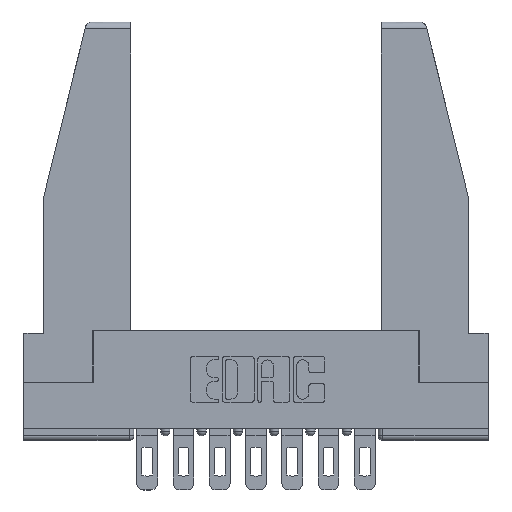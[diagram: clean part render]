
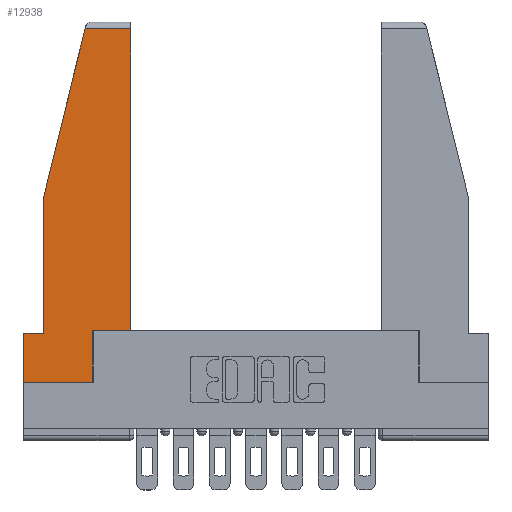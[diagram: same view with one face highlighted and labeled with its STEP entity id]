
A CAD part, top view. The second image highlights one B-rep face of the part: STEP entity #12938.
In plain terms, the highlighted planar face has unit normal (0, 0, 1).
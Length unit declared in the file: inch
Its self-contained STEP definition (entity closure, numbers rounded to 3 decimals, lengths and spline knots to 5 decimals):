
#325 = LINE ( 'NONE', #12492, #6050 ) ;
#330 = EDGE_CURVE ( 'NONE', #11068, #5160, #11624, .T. ) ;
#510 = ORIENTED_EDGE ( 'NONE', *, *, #4445, .T. ) ;
#1410 = LINE ( 'NONE', #4657, #11373 ) ;
#1658 = CARTESIAN_POINT ( 'NONE',  ( 0., 0.21, 0. ) ) ;
#1961 = VERTEX_POINT ( 'NONE', #8863 ) ;
#2006 = DIRECTION ( 'NONE',  ( -0.239, -0.971, 0. ) ) ;
#2107 = DIRECTION ( 'NONE',  ( 0., -1., 0. ) ) ;
#2191 = CARTESIAN_POINT ( 'NONE',  ( 0.086, 0.8, 0. ) ) ;
#2214 = LINE ( 'NONE', #5121, #5008 ) ;
#2404 = EDGE_CURVE ( 'NONE', #5160, #3727, #9088, .T. ) ;
#2433 = VECTOR ( 'NONE', #8961, 39.37008 ) ;
#2549 = CARTESIAN_POINT ( 'NONE',  ( 0.461, 1.52, 0. ) ) ;
#2828 = EDGE_CURVE ( 'NONE', #8333, #1961, #1410, .T. ) ;
#2837 = AXIS2_PLACEMENT_3D ( 'NONE', #11134, #10031, #13263 ) ;
#2905 = DIRECTION ( 'NONE',  ( -1., 0., 0. ) ) ;
#2972 = EDGE_CURVE ( 'NONE', #5855, #11068, #2214, .T. ) ;
#3239 = DIRECTION ( 'NONE',  ( 0., 1., 0. ) ) ;
#3332 = LINE ( 'NONE', #4401, #3661 ) ;
#3661 = VECTOR ( 'NONE', #3239, 39.37008 ) ;
#3727 = VERTEX_POINT ( 'NONE', #4816 ) ;
#3913 = EDGE_CURVE ( 'NONE', #1961, #5855, #3332, .T. ) ;
#4401 = CARTESIAN_POINT ( 'NONE',  ( 0.297, 0., 0. ) ) ;
#4445 = EDGE_CURVE ( 'NONE', #9360, #13013, #13496, .T. ) ;
#4657 = CARTESIAN_POINT ( 'NONE',  ( 0., 0., 0. ) ) ;
#4816 = CARTESIAN_POINT ( 'NONE',  ( 0.2636, 1.52, 0. ) ) ;
#4980 = DIRECTION ( 'NONE',  ( 1., 0., 0. ) ) ;
#5008 = VECTOR ( 'NONE', #4980, 39.37008 ) ;
#5121 = CARTESIAN_POINT ( 'NONE',  ( 0.297, 0.223, 0. ) ) ;
#5160 = VERTEX_POINT ( 'NONE', #2549 ) ;
#5519 = VECTOR ( 'NONE', #2905, 39.37008 ) ;
#5855 = VERTEX_POINT ( 'NONE', #6613 ) ;
#6015 = EDGE_CURVE ( 'NONE', #13013, #8176, #325, .T. ) ;
#6029 = CARTESIAN_POINT ( 'NONE',  ( 0.086, 0.21, 0. ) ) ;
#6050 = VECTOR ( 'NONE', #10335, 39.37008 ) ;
#6460 = EDGE_CURVE ( 'NONE', #8176, #8333, #8006, .T. ) ;
#6544 = ORIENTED_EDGE ( 'NONE', *, *, #6015, .T. ) ;
#6613 = CARTESIAN_POINT ( 'NONE',  ( 0.297, 0.223, 0. ) ) ;
#6689 = EDGE_CURVE ( 'NONE', #3727, #9360, #11585, .T. ) ;
#6868 = PLANE ( 'NONE',  #2837 ) ;
#7839 = EDGE_LOOP ( 'NONE', ( #8641, #9992, #8361, #510, #6544, #10832, #12906, #13343, #13008 ) ) ;
#8006 = LINE ( 'NONE', #1658, #2433 ) ;
#8176 = VERTEX_POINT ( 'NONE', #8384 ) ;
#8222 = FACE_OUTER_BOUND ( 'NONE', #7839, .T. ) ;
#8333 = VERTEX_POINT ( 'NONE', #9545 ) ;
#8361 = ORIENTED_EDGE ( 'NONE', *, *, #6689, .T. ) ;
#8384 = CARTESIAN_POINT ( 'NONE',  ( 0., 0.21, 0. ) ) ;
#8641 = ORIENTED_EDGE ( 'NONE', *, *, #330, .T. ) ;
#8863 = CARTESIAN_POINT ( 'NONE',  ( 0.297, 0., 0. ) ) ;
#8961 = DIRECTION ( 'NONE',  ( 0., -1., 0. ) ) ;
#9088 = LINE ( 'NONE', #9269, #5519 ) ;
#9269 = CARTESIAN_POINT ( 'NONE',  ( 0., 1.52, 0. ) ) ;
#9360 = VERTEX_POINT ( 'NONE', #9475 ) ;
#9475 = CARTESIAN_POINT ( 'NONE',  ( 0.086, 0.8, 0. ) ) ;
#9545 = CARTESIAN_POINT ( 'NONE',  ( 0., 0., 0. ) ) ;
#9992 = ORIENTED_EDGE ( 'NONE', *, *, #2404, .T. ) ;
#10031 = DIRECTION ( 'NONE',  ( 0., 0., 1. ) ) ;
#10335 = DIRECTION ( 'NONE',  ( -1., 0., 0. ) ) ;
#10365 = VECTOR ( 'NONE', #2107, 39.37008 ) ;
#10469 = CARTESIAN_POINT ( 'NONE',  ( 0.271, 1.55, 0. ) ) ;
#10832 = ORIENTED_EDGE ( 'NONE', *, *, #6460, .T. ) ;
#11015 = DIRECTION ( 'NONE',  ( 0., 1., 0. ) ) ;
#11068 = VERTEX_POINT ( 'NONE', #11638 ) ;
#11108 = VECTOR ( 'NONE', #11015, 39.37008 ) ;
#11134 = CARTESIAN_POINT ( 'NONE',  ( 0., 0., 0. ) ) ;
#11373 = VECTOR ( 'NONE', #12001, 39.37008 ) ;
#11585 = LINE ( 'NONE', #10469, #11905 ) ;
#11624 = LINE ( 'NONE', #12032, #11108 ) ;
#11638 = CARTESIAN_POINT ( 'NONE',  ( 0.461, 0.223, 0. ) ) ;
#11905 = VECTOR ( 'NONE', #2006, 39.37008 ) ;
#12001 = DIRECTION ( 'NONE',  ( 1., 0., 0. ) ) ;
#12032 = CARTESIAN_POINT ( 'NONE',  ( 0.461, 0.223, 0. ) ) ;
#12492 = CARTESIAN_POINT ( 'NONE',  ( 0., 0.21, 0. ) ) ;
#12906 = ORIENTED_EDGE ( 'NONE', *, *, #2828, .T. ) ;
#12938 = ADVANCED_FACE ( 'NONE', ( #8222 ), #6868, .T. ) ;
#13008 = ORIENTED_EDGE ( 'NONE', *, *, #2972, .T. ) ;
#13013 = VERTEX_POINT ( 'NONE', #6029 ) ;
#13263 = DIRECTION ( 'NONE',  ( 1., 0., 0. ) ) ;
#13343 = ORIENTED_EDGE ( 'NONE', *, *, #3913, .T. ) ;
#13496 = LINE ( 'NONE', #2191, #10365 ) ;
